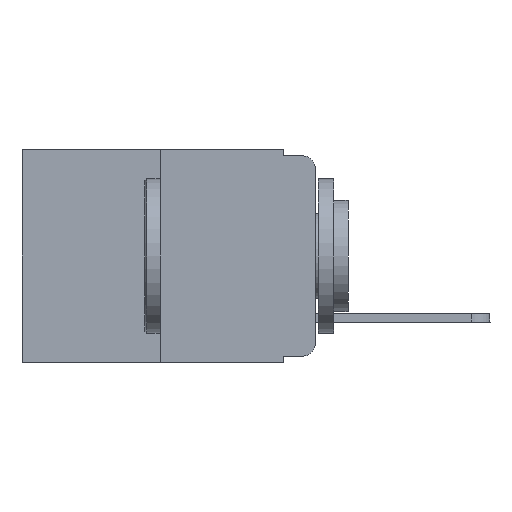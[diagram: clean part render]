
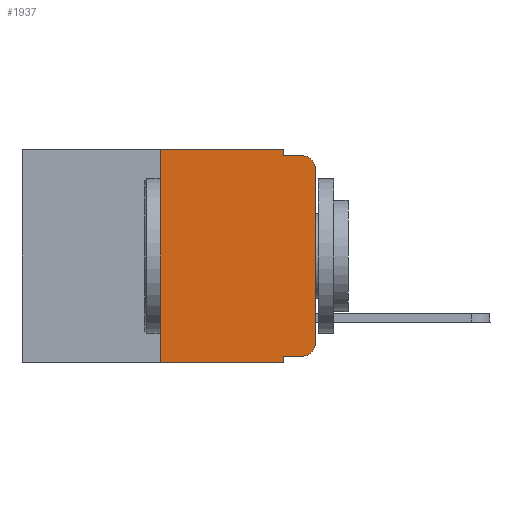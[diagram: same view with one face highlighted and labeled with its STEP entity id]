
A CAD part, left-side view. The second image highlights one B-rep face of the part: STEP entity #1937.
In plain terms, the highlighted planar face has unit normal (-1, 0, 0).
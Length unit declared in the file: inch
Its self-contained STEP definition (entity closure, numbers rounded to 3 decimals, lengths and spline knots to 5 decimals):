
#32 = LINE ( 'NONE', #5640, #12467 ) ;
#40 = CARTESIAN_POINT ( 'NONE',  ( 0., 0.473, 0. ) ) ;
#56 = CARTESIAN_POINT ( 'NONE',  ( 0., 0.02, -0.03 ) ) ;
#151 = AXIS2_PLACEMENT_3D ( 'NONE', #6501, #13142, #2113 ) ;
#245 = EDGE_CURVE ( 'NONE', #11673, #13612, #6624, .T. ) ;
#396 = VERTEX_POINT ( 'NONE', #9819 ) ;
#488 = VECTOR ( 'NONE', #6580, 39.37008 ) ;
#578 = CARTESIAN_POINT ( 'NONE',  ( 0., 0., -0.313 ) ) ;
#772 = ORIENTED_EDGE ( 'NONE', *, *, #8539, .T. ) ;
#813 = VECTOR ( 'NONE', #1127, 39.37008 ) ;
#1127 = DIRECTION ( 'NONE',  ( 0., 0., 1. ) ) ;
#1577 = CARTESIAN_POINT ( 'NONE',  ( 0., 0.051, -0.333 ) ) ;
#1728 = EDGE_CURVE ( 'NONE', #6823, #4477, #32, .T. ) ;
#1795 = CARTESIAN_POINT ( 'NONE',  ( 0., 0.02, -0.313 ) ) ;
#1919 = PLANE ( 'NONE',  #151 ) ;
#1937 = ADVANCED_FACE ( 'NONE', ( #5182 ), #1919, .F. ) ;
#2057 = DIRECTION ( 'NONE',  ( -1., 0., 0. ) ) ;
#2113 = DIRECTION ( 'NONE',  ( 0., 0., -1. ) ) ;
#2631 = EDGE_CURVE ( 'NONE', #6855, #4326, #12405, .T. ) ;
#2998 = EDGE_CURVE ( 'NONE', #4477, #6855, #3409, .T. ) ;
#3267 = DIRECTION ( 'NONE',  ( 0., 0., -1. ) ) ;
#3278 = LINE ( 'NONE', #10971, #11733 ) ;
#3367 = CARTESIAN_POINT ( 'NONE',  ( 0., 0.02, -0.01 ) ) ;
#3409 = LINE ( 'NONE', #40, #488 ) ;
#3478 = CARTESIAN_POINT ( 'NONE',  ( 0., 0.25, -0.343 ) ) ;
#3952 = ORIENTED_EDGE ( 'NONE', *, *, #8073, .F. ) ;
#4054 = ORIENTED_EDGE ( 'NONE', *, *, #9954, .T. ) ;
#4106 = LINE ( 'NONE', #7329, #6904 ) ;
#4127 = ORIENTED_EDGE ( 'NONE', *, *, #2631, .F. ) ;
#4326 = VERTEX_POINT ( 'NONE', #6849 ) ;
#4404 = DIRECTION ( 'NONE',  ( 0., -1., 0. ) ) ;
#4477 = VERTEX_POINT ( 'NONE', #9376 ) ;
#4517 = LINE ( 'NONE', #5616, #13021 ) ;
#4717 = LINE ( 'NONE', #12388, #8548 ) ;
#5182 = FACE_OUTER_BOUND ( 'NONE', #11981, .T. ) ;
#5256 = CARTESIAN_POINT ( 'NONE',  ( 0., 0.02, -0.333 ) ) ;
#5322 = CIRCLE ( 'NONE', #9804, 0.02 ) ;
#5616 = CARTESIAN_POINT ( 'NONE',  ( 0., 0.051, -0.333 ) ) ;
#5640 = CARTESIAN_POINT ( 'NONE',  ( 0., 0.25, 0. ) ) ;
#5991 = ORIENTED_EDGE ( 'NONE', *, *, #14287, .F. ) ;
#6356 = DIRECTION ( 'NONE',  ( 0., 0., -1. ) ) ;
#6501 = CARTESIAN_POINT ( 'NONE',  ( 0., 0.473, 0. ) ) ;
#6560 = DIRECTION ( 'NONE',  ( 0., -1., 0. ) ) ;
#6580 = DIRECTION ( 'NONE',  ( 0., -1., 0. ) ) ;
#6582 = CARTESIAN_POINT ( 'NONE',  ( 0., 0.051, 0. ) ) ;
#6624 = CIRCLE ( 'NONE', #8445, 0.02 ) ;
#6651 = CARTESIAN_POINT ( 'NONE',  ( 0., 0.051, 0. ) ) ;
#6658 = ORIENTED_EDGE ( 'NONE', *, *, #7274, .T. ) ;
#6708 = CARTESIAN_POINT ( 'NONE',  ( 0., 0., 0. ) ) ;
#6823 = VERTEX_POINT ( 'NONE', #3478 ) ;
#6849 = CARTESIAN_POINT ( 'NONE',  ( 0., 0.051, -0.01 ) ) ;
#6855 = VERTEX_POINT ( 'NONE', #6651 ) ;
#6904 = VECTOR ( 'NONE', #8465, 39.37008 ) ;
#7274 = EDGE_CURVE ( 'NONE', #396, #9302, #5322, .T. ) ;
#7329 = CARTESIAN_POINT ( 'NONE',  ( 0., 0.051, 0. ) ) ;
#7864 = ORIENTED_EDGE ( 'NONE', *, *, #1728, .F. ) ;
#7865 = ORIENTED_EDGE ( 'NONE', *, *, #2998, .F. ) ;
#8073 = EDGE_CURVE ( 'NONE', #4326, #9302, #4717, .T. ) ;
#8445 = AXIS2_PLACEMENT_3D ( 'NONE', #1795, #13000, #6356 ) ;
#8465 = DIRECTION ( 'NONE',  ( 0., 0., -1. ) ) ;
#8539 = EDGE_CURVE ( 'NONE', #6823, #13747, #3278, .T. ) ;
#8548 = VECTOR ( 'NONE', #9109, 39.37008 ) ;
#9109 = DIRECTION ( 'NONE',  ( 0., -1., 0. ) ) ;
#9302 = VERTEX_POINT ( 'NONE', #3367 ) ;
#9376 = CARTESIAN_POINT ( 'NONE',  ( 0., 0.25, 0. ) ) ;
#9804 = AXIS2_PLACEMENT_3D ( 'NONE', #56, #2057, #11005 ) ;
#9819 = CARTESIAN_POINT ( 'NONE',  ( 0., 0., -0.03 ) ) ;
#9954 = EDGE_CURVE ( 'NONE', #13612, #396, #9955, .T. ) ;
#9955 = LINE ( 'NONE', #6708, #813 ) ;
#10340 = ORIENTED_EDGE ( 'NONE', *, *, #245, .T. ) ;
#10722 = VERTEX_POINT ( 'NONE', #1577 ) ;
#10971 = CARTESIAN_POINT ( 'NONE',  ( 0., 0.473, -0.343 ) ) ;
#11005 = DIRECTION ( 'NONE',  ( 0., 0., -1. ) ) ;
#11529 = VECTOR ( 'NONE', #3267, 39.37008 ) ;
#11673 = VERTEX_POINT ( 'NONE', #5256 ) ;
#11733 = VECTOR ( 'NONE', #6560, 39.37008 ) ;
#11981 = EDGE_LOOP ( 'NONE', ( #4054, #6658, #3952, #4127, #7865, #7864, #772, #5991, #12747, #10340 ) ) ;
#12228 = DIRECTION ( 'NONE',  ( 0., 0., 1. ) ) ;
#12388 = CARTESIAN_POINT ( 'NONE',  ( 0., 0.051, -0.01 ) ) ;
#12405 = LINE ( 'NONE', #6582, #11529 ) ;
#12435 = EDGE_CURVE ( 'NONE', #10722, #11673, #4517, .T. ) ;
#12467 = VECTOR ( 'NONE', #12228, 39.37008 ) ;
#12747 = ORIENTED_EDGE ( 'NONE', *, *, #12435, .T. ) ;
#12820 = CARTESIAN_POINT ( 'NONE',  ( 0., 0.051, -0.343 ) ) ;
#13000 = DIRECTION ( 'NONE',  ( -1., 0., 0. ) ) ;
#13021 = VECTOR ( 'NONE', #4404, 39.37008 ) ;
#13142 = DIRECTION ( 'NONE',  ( 1., 0., 0. ) ) ;
#13612 = VERTEX_POINT ( 'NONE', #578 ) ;
#13747 = VERTEX_POINT ( 'NONE', #12820 ) ;
#14287 = EDGE_CURVE ( 'NONE', #10722, #13747, #4106, .T. ) ;
